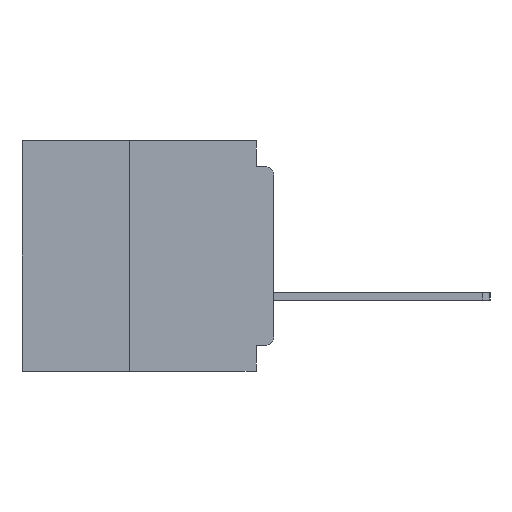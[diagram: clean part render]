
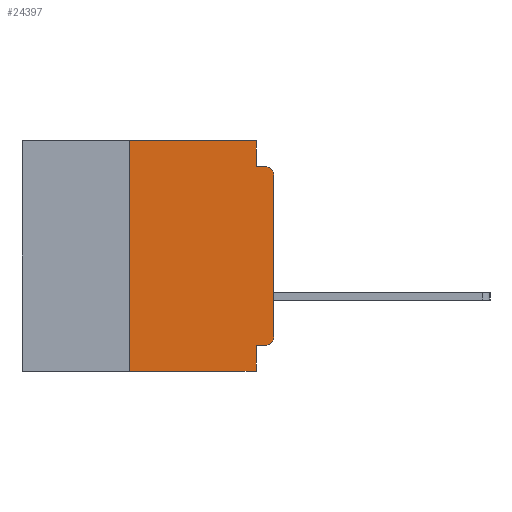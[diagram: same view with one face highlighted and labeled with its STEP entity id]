
A CAD part, left-side view. The second image highlights one B-rep face of the part: STEP entity #24397.
In plain terms, the highlighted planar face has unit normal (-1, 0, 0).
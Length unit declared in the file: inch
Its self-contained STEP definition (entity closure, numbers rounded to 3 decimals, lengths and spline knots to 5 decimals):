
#1101 = CIRCLE ( 'NONE', #36020, 0.015 ) ;
#1710 = DIRECTION ( 'NONE',  ( 0., -1., 0. ) ) ;
#3695 = EDGE_CURVE ( 'NONE', #56947, #19914, #23816, .T. ) ;
#3781 = EDGE_CURVE ( 'NONE', #56869, #30436, #4916, .T. ) ;
#4032 = DIRECTION ( 'NONE',  ( 0., 0., -1. ) ) ;
#4709 = CIRCLE ( 'NONE', #6521, 0.015 ) ;
#4821 = CARTESIAN_POINT ( 'NONE',  ( 0., 0.25, -0.4 ) ) ;
#4916 = LINE ( 'NONE', #63984, #31098 ) ;
#5091 = CARTESIAN_POINT ( 'NONE',  ( 0., 0.25, 0. ) ) ;
#6286 = DIRECTION ( 'NONE',  ( 0., 0., 1. ) ) ;
#6521 = AXIS2_PLACEMENT_3D ( 'NONE', #66298, #35343, #4032 ) ;
#6540 = DIRECTION ( 'NONE',  ( 0., 0., -1. ) ) ;
#8982 = EDGE_CURVE ( 'NONE', #30436, #17608, #34629, .T. ) ;
#9510 = ORIENTED_EDGE ( 'NONE', *, *, #3695, .T. ) ;
#9602 = LINE ( 'NONE', #51320, #21974 ) ;
#9863 = VECTOR ( 'NONE', #6286, 39.37008 ) ;
#9874 = DIRECTION ( 'NONE',  ( 0., 0., -1. ) ) ;
#10004 = CARTESIAN_POINT ( 'NONE',  ( 0., 0.031, -0.4 ) ) ;
#10111 = DIRECTION ( 'NONE',  ( 0., 0., 1. ) ) ;
#10298 = LINE ( 'NONE', #31317, #22643 ) ;
#11096 = FACE_OUTER_BOUND ( 'NONE', #64030, .T. ) ;
#13305 = EDGE_CURVE ( 'NONE', #17608, #54850, #10298, .T. ) ;
#13633 = CARTESIAN_POINT ( 'NONE',  ( 0., 0.25, -0.4 ) ) ;
#14971 = ORIENTED_EDGE ( 'NONE', *, *, #45611, .F. ) ;
#15531 = ORIENTED_EDGE ( 'NONE', *, *, #38452, .T. ) ;
#15871 = CARTESIAN_POINT ( 'NONE',  ( 0., 0.031, -0.4 ) ) ;
#16497 = CARTESIAN_POINT ( 'NONE',  ( 0., 0., -0.06 ) ) ;
#17074 = LINE ( 'NONE', #10004, #30875 ) ;
#17608 = VERTEX_POINT ( 'NONE', #65462 ) ;
#19370 = DIRECTION ( 'NONE',  ( 0., 1., 0. ) ) ;
#19914 = VERTEX_POINT ( 'NONE', #16497 ) ;
#21974 = VECTOR ( 'NONE', #25444, 39.37008 ) ;
#22643 = VECTOR ( 'NONE', #26124, 39.37008 ) ;
#23786 = ORIENTED_EDGE ( 'NONE', *, *, #8982, .F. ) ;
#23816 = LINE ( 'NONE', #63109, #9863 ) ;
#24397 = ADVANCED_FACE ( 'NONE', ( #11096 ), #53213, .F. ) ;
#25444 = DIRECTION ( 'NONE',  ( 0., -1., 0. ) ) ;
#26124 = DIRECTION ( 'NONE',  ( 0., -1., 0. ) ) ;
#26665 = VECTOR ( 'NONE', #10111, 39.37008 ) ;
#28205 = DIRECTION ( 'NONE',  ( -1., 0., 0. ) ) ;
#29515 = LINE ( 'NONE', #45267, #40077 ) ;
#29775 = VECTOR ( 'NONE', #9874, 39.37008 ) ;
#30436 = VERTEX_POINT ( 'NONE', #42131 ) ;
#30875 = VECTOR ( 'NONE', #51661, 39.37008 ) ;
#30885 = CARTESIAN_POINT ( 'NONE',  ( 0., 0.031, 0. ) ) ;
#31098 = VECTOR ( 'NONE', #1710, 39.37008 ) ;
#31100 = ORIENTED_EDGE ( 'NONE', *, *, #57964, .T. ) ;
#31317 = CARTESIAN_POINT ( 'NONE',  ( 0., 0., -0.045 ) ) ;
#34546 = CARTESIAN_POINT ( 'NONE',  ( 0., 0.015, -0.045 ) ) ;
#34629 = LINE ( 'NONE', #30885, #29775 ) ;
#35343 = DIRECTION ( 'NONE',  ( -1., 0., 0. ) ) ;
#36020 = AXIS2_PLACEMENT_3D ( 'NONE', #59194, #28205, #64386 ) ;
#36776 = AXIS2_PLACEMENT_3D ( 'NONE', #42820, #37837, #6540 ) ;
#37837 = DIRECTION ( 'NONE',  ( 1., 0., 0. ) ) ;
#38314 = VERTEX_POINT ( 'NONE', #13633 ) ;
#38452 = EDGE_CURVE ( 'NONE', #38314, #60779, #9602, .T. ) ;
#38848 = VERTEX_POINT ( 'NONE', #39276 ) ;
#39276 = CARTESIAN_POINT ( 'NONE',  ( 0., 0.031, -0.355 ) ) ;
#40077 = VECTOR ( 'NONE', #19370, 39.37008 ) ;
#40479 = LINE ( 'NONE', #4821, #26665 ) ;
#40695 = ORIENTED_EDGE ( 'NONE', *, *, #62208, .T. ) ;
#41006 = ORIENTED_EDGE ( 'NONE', *, *, #43273, .F. ) ;
#41025 = CARTESIAN_POINT ( 'NONE',  ( 0., 0.015, -0.355 ) ) ;
#42131 = CARTESIAN_POINT ( 'NONE',  ( 0., 0.031, 0. ) ) ;
#42820 = CARTESIAN_POINT ( 'NONE',  ( 0., 0.437, 0. ) ) ;
#42845 = ORIENTED_EDGE ( 'NONE', *, *, #13305, .F. ) ;
#43273 = EDGE_CURVE ( 'NONE', #58023, #38848, #29515, .T. ) ;
#45267 = CARTESIAN_POINT ( 'NONE',  ( 0., 0., -0.355 ) ) ;
#45611 = EDGE_CURVE ( 'NONE', #38848, #60779, #17074, .T. ) ;
#46762 = EDGE_CURVE ( 'NONE', #38314, #56869, #40479, .T. ) ;
#47554 = CARTESIAN_POINT ( 'NONE',  ( 0., 0., -0.34 ) ) ;
#51320 = CARTESIAN_POINT ( 'NONE',  ( 0., 0.437, -0.4 ) ) ;
#51661 = DIRECTION ( 'NONE',  ( 0., 0., -1. ) ) ;
#53213 = PLANE ( 'NONE',  #36776 ) ;
#54850 = VERTEX_POINT ( 'NONE', #34546 ) ;
#56591 = ORIENTED_EDGE ( 'NONE', *, *, #3781, .F. ) ;
#56869 = VERTEX_POINT ( 'NONE', #5091 ) ;
#56947 = VERTEX_POINT ( 'NONE', #47554 ) ;
#57964 = EDGE_CURVE ( 'NONE', #19914, #54850, #4709, .T. ) ;
#58023 = VERTEX_POINT ( 'NONE', #41025 ) ;
#59194 = CARTESIAN_POINT ( 'NONE',  ( 0., 0.015, -0.34 ) ) ;
#60779 = VERTEX_POINT ( 'NONE', #15871 ) ;
#62208 = EDGE_CURVE ( 'NONE', #58023, #56947, #1101, .T. ) ;
#63109 = CARTESIAN_POINT ( 'NONE',  ( 0., 0., 0. ) ) ;
#63587 = ORIENTED_EDGE ( 'NONE', *, *, #46762, .F. ) ;
#63984 = CARTESIAN_POINT ( 'NONE',  ( 0., 0.437, 0. ) ) ;
#64030 = EDGE_LOOP ( 'NONE', ( #9510, #31100, #42845, #23786, #56591, #63587, #15531, #14971, #41006, #40695 ) ) ;
#64386 = DIRECTION ( 'NONE',  ( 0., 0., -1. ) ) ;
#65462 = CARTESIAN_POINT ( 'NONE',  ( 0., 0.031, -0.045 ) ) ;
#66298 = CARTESIAN_POINT ( 'NONE',  ( 0., 0.015, -0.06 ) ) ;
